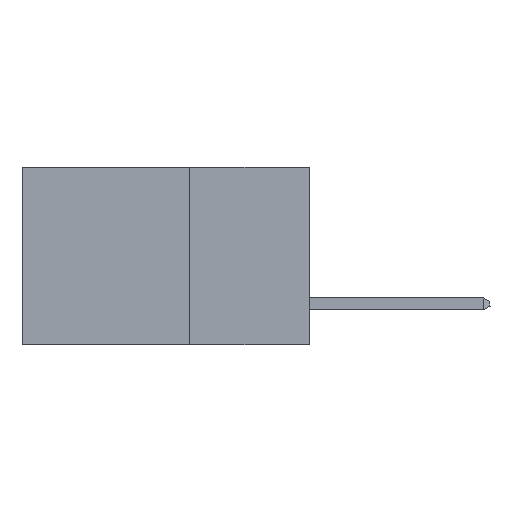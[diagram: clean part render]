
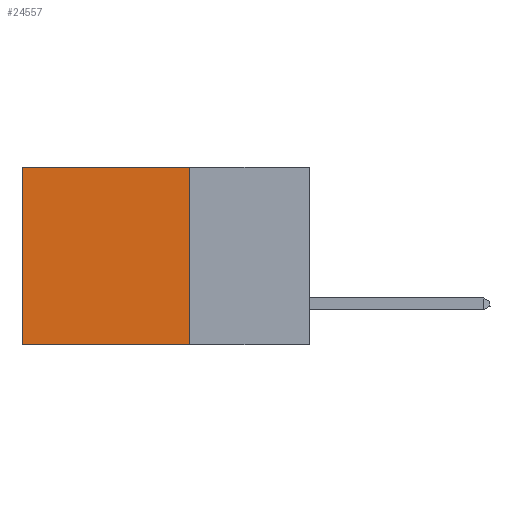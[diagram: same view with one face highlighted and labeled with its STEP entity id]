
A CAD part, left-side view. The second image highlights one B-rep face of the part: STEP entity #24557.
In plain terms, the highlighted planar face has unit normal (-1, 0, 0).
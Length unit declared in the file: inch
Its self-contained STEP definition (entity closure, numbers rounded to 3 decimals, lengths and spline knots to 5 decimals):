
#718 = CARTESIAN_POINT ( 'NONE',  ( 0.2875, 0.6, 0. ) ) ;
#2665 = CARTESIAN_POINT ( 'NONE',  ( 0.2875, 0.6, -0.37 ) ) ;
#3477 = VERTEX_POINT ( 'NONE', #18182 ) ;
#4231 = EDGE_CURVE ( 'NONE', #34806, #21750, #32253, .T. ) ;
#4889 = CARTESIAN_POINT ( 'NONE',  ( 0.2875, 0.25, 0. ) ) ;
#8230 = VECTOR ( 'NONE', #14776, 39.37008 ) ;
#8835 = EDGE_CURVE ( 'NONE', #36908, #3477, #26431, .T. ) ;
#13638 = LINE ( 'NONE', #4889, #21791 ) ;
#14347 = DIRECTION ( 'NONE',  ( 0., 0., -1. ) ) ;
#14405 = PLANE ( 'NONE',  #41110 ) ;
#14776 = DIRECTION ( 'NONE',  ( 0., 1., 0. ) ) ;
#15089 = ORIENTED_EDGE ( 'NONE', *, *, #24148, .T. ) ;
#15924 = CARTESIAN_POINT ( 'NONE',  ( 0.2875, 0.25, 0. ) ) ;
#18182 = CARTESIAN_POINT ( 'NONE',  ( 0.2875, 0.25, -0.37 ) ) ;
#21521 = DIRECTION ( 'NONE',  ( 0., 0., -1. ) ) ;
#21750 = VERTEX_POINT ( 'NONE', #2665 ) ;
#21791 = VECTOR ( 'NONE', #32772, 39.37008 ) ;
#23758 = VECTOR ( 'NONE', #21521, 39.37008 ) ;
#24148 = EDGE_CURVE ( 'NONE', #36908, #34806, #13638, .T. ) ;
#24450 = EDGE_LOOP ( 'NONE', ( #44528, #24919, #25287, #15089 ) ) ;
#24557 = ADVANCED_FACE ( 'NONE', ( #38145 ), #14405, .F. ) ;
#24919 = ORIENTED_EDGE ( 'NONE', *, *, #30421, .F. ) ;
#24990 = DIRECTION ( 'NONE',  ( 0., 0., -1. ) ) ;
#25075 = CARTESIAN_POINT ( 'NONE',  ( 0.2875, 0.25, 0. ) ) ;
#25287 = ORIENTED_EDGE ( 'NONE', *, *, #8835, .F. ) ;
#26431 = LINE ( 'NONE', #33222, #23758 ) ;
#28220 = CARTESIAN_POINT ( 'NONE',  ( 0.2875, 0.6, 0. ) ) ;
#30421 = EDGE_CURVE ( 'NONE', #3477, #21750, #41002, .T. ) ;
#32253 = LINE ( 'NONE', #28220, #40518 ) ;
#32772 = DIRECTION ( 'NONE',  ( 0., 1., 0. ) ) ;
#33222 = CARTESIAN_POINT ( 'NONE',  ( 0.2875, 0.25, 0. ) ) ;
#34806 = VERTEX_POINT ( 'NONE', #718 ) ;
#35640 = CARTESIAN_POINT ( 'NONE',  ( 0.2875, 0.25, -0.37 ) ) ;
#36908 = VERTEX_POINT ( 'NONE', #15924 ) ;
#38145 = FACE_OUTER_BOUND ( 'NONE', #24450, .T. ) ;
#40518 = VECTOR ( 'NONE', #14347, 39.37008 ) ;
#41002 = LINE ( 'NONE', #35640, #8230 ) ;
#41110 = AXIS2_PLACEMENT_3D ( 'NONE', #25075, #43963, #24990 ) ;
#43963 = DIRECTION ( 'NONE',  ( 1., 0., 0. ) ) ;
#44528 = ORIENTED_EDGE ( 'NONE', *, *, #4231, .T. ) ;
